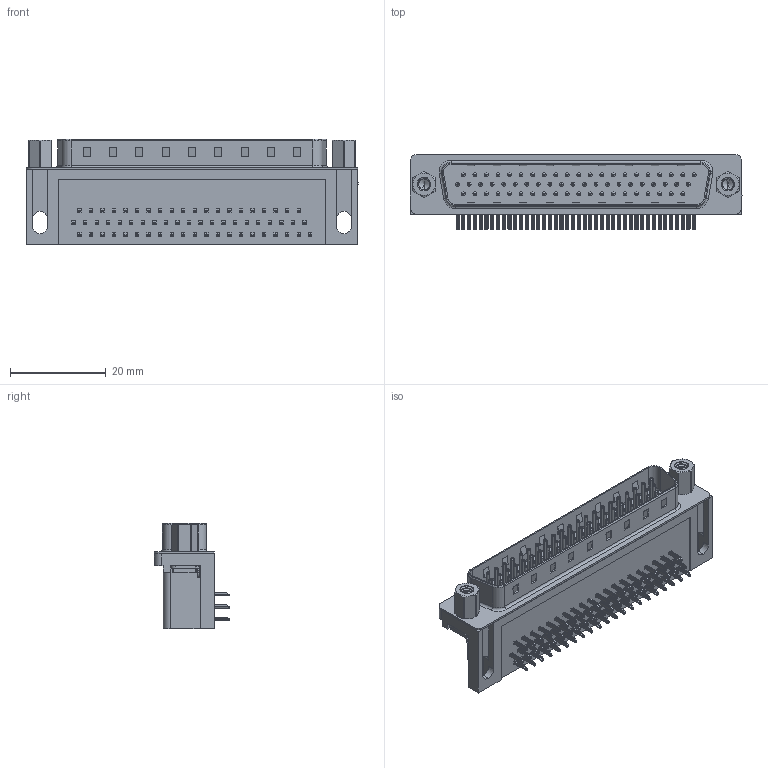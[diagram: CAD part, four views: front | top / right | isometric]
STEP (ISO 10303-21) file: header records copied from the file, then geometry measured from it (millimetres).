
FILE_DESCRIPTION (( 'STEP AP203' ), '1' );
FILE_NAME ('633-062-663-003.STEP', '2018-09-07T22:30:49', ( '' ), ( '' ), 'SwSTEP 2.0', 'SolidWorks 2016', '' );
FILE_SCHEMA (( 'CONFIG_CONTROL_DESIGN' ));
Length unit declared in the file: millimetre
Products named in the file (9): 633 4-40 Threaded Rivet; 633 4-40 Hex Standoff; 633-062-663-003; 633 Housing_62 Contact; 633 Shell_62 Contact; 633 Contact Bottom; 633 Contact Middle; 633 Contact Top; 633 Non Board Mount
Assembly tree (70 placements, depth 2):
  633-062-663-003
    633 Housing_62 Contact
    633 Shell_62 Contact
    633 Contact Bottom  x20
    633 Contact Middle  x21
    633 Contact Top  x21
    633 Non Board Mount  x2
    633 4-40 Threaded Rivet  x2
    633 4-40 Hex Standoff  x2
Bounding box: 69.4 x 15.73 x 22.1 mm (x, y, z)
Volume: 11209.3 mm3; surface area: 13635.1 mm2
Topology: 70 solids, 70 shells, 5192 faces, 12802 edges, 7881 vertices
Faces by surface type: plane 3235, cylinder 1502, torus 403, cone 34, bspline 18
Entity records: 39416 total; most frequent: CARTESIAN_POINT 9945, DIRECTION 5624, ORIENTED_EDGE 5450, EDGE_CURVE 2725, LINE 1914, VECTOR 1914, AXIS2_PLACEMENT_3D 1855, VERTEX_POINT 1761
